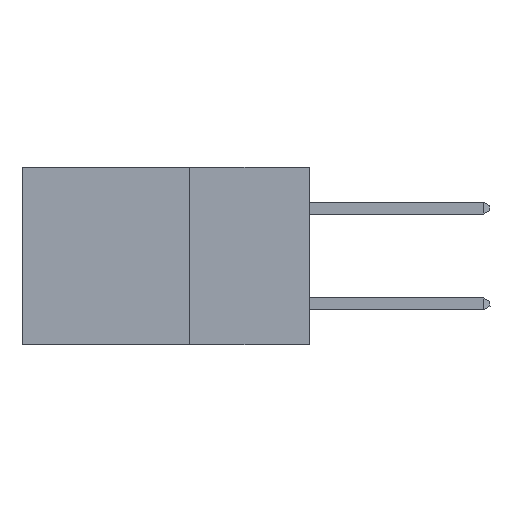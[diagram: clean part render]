
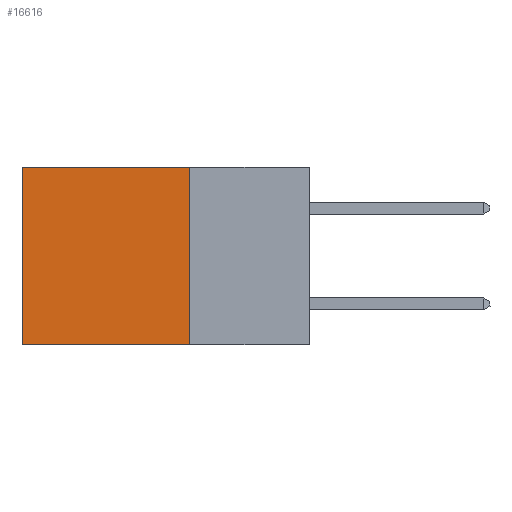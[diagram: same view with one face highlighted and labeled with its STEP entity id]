
A CAD part, left-side view. The second image highlights one B-rep face of the part: STEP entity #16616.
In plain terms, the highlighted planar face has unit normal (-1, 0, 0).
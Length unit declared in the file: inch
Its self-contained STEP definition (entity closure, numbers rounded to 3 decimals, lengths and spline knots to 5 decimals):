
#476 = VECTOR ( 'NONE', #21790, 39.37008 ) ;
#1235 = LINE ( 'NONE', #16809, #4710 ) ;
#2301 = ORIENTED_EDGE ( 'NONE', *, *, #12996, .F. ) ;
#2793 = VERTEX_POINT ( 'NONE', #7564 ) ;
#3127 = VECTOR ( 'NONE', #18019, 39.37008 ) ;
#3504 = AXIS2_PLACEMENT_3D ( 'NONE', #17865, #9478, #21179 ) ;
#3585 = LINE ( 'NONE', #17374, #20430 ) ;
#3774 = FACE_OUTER_BOUND ( 'NONE', #7325, .T. ) ;
#3803 = VERTEX_POINT ( 'NONE', #6621 ) ;
#3810 = CARTESIAN_POINT ( 'NONE',  ( 0.2875, 0.6, -0.37 ) ) ;
#3904 = DIRECTION ( 'NONE',  ( 0., 1., 0. ) ) ;
#4710 = VECTOR ( 'NONE', #15107, 39.37008 ) ;
#6520 = ORIENTED_EDGE ( 'NONE', *, *, #11560, .T. ) ;
#6621 = CARTESIAN_POINT ( 'NONE',  ( 0.2875, 0.25, -0.37 ) ) ;
#7325 = EDGE_LOOP ( 'NONE', ( #7346, #2301, #21296, #6520 ) ) ;
#7346 = ORIENTED_EDGE ( 'NONE', *, *, #18501, .T. ) ;
#7564 = CARTESIAN_POINT ( 'NONE',  ( 0.2875, 0.6, 0. ) ) ;
#9478 = DIRECTION ( 'NONE',  ( 1., 0., 0. ) ) ;
#11560 = EDGE_CURVE ( 'NONE', #13150, #2793, #1235, .T. ) ;
#12155 = LINE ( 'NONE', #16279, #3127 ) ;
#12996 = EDGE_CURVE ( 'NONE', #3803, #18656, #3585, .T. ) ;
#13150 = VERTEX_POINT ( 'NONE', #19504 ) ;
#14457 = PLANE ( 'NONE',  #3504 ) ;
#15050 = CARTESIAN_POINT ( 'NONE',  ( 0.2875, 0.6, 0. ) ) ;
#15107 = DIRECTION ( 'NONE',  ( 0., 1., 0. ) ) ;
#16279 = CARTESIAN_POINT ( 'NONE',  ( 0.2875, 0.25, 0. ) ) ;
#16616 = ADVANCED_FACE ( 'NONE', ( #3774 ), #14457, .F. ) ;
#16809 = CARTESIAN_POINT ( 'NONE',  ( 0.2875, 0.25, 0. ) ) ;
#17374 = CARTESIAN_POINT ( 'NONE',  ( 0.2875, 0.25, -0.37 ) ) ;
#17865 = CARTESIAN_POINT ( 'NONE',  ( 0.2875, 0.25, 0. ) ) ;
#18019 = DIRECTION ( 'NONE',  ( 0., 0., -1. ) ) ;
#18453 = LINE ( 'NONE', #15050, #476 ) ;
#18501 = EDGE_CURVE ( 'NONE', #2793, #18656, #18453, .T. ) ;
#18656 = VERTEX_POINT ( 'NONE', #3810 ) ;
#19504 = CARTESIAN_POINT ( 'NONE',  ( 0.2875, 0.25, 0. ) ) ;
#20430 = VECTOR ( 'NONE', #3904, 39.37008 ) ;
#20690 = EDGE_CURVE ( 'NONE', #13150, #3803, #12155, .T. ) ;
#21179 = DIRECTION ( 'NONE',  ( 0., 0., -1. ) ) ;
#21296 = ORIENTED_EDGE ( 'NONE', *, *, #20690, .F. ) ;
#21790 = DIRECTION ( 'NONE',  ( 0., 0., -1. ) ) ;
